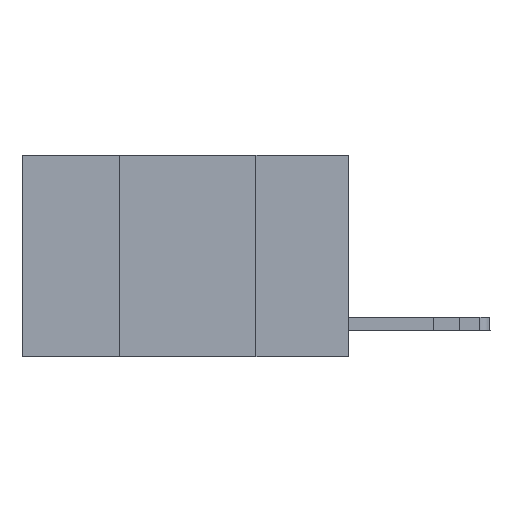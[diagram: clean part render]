
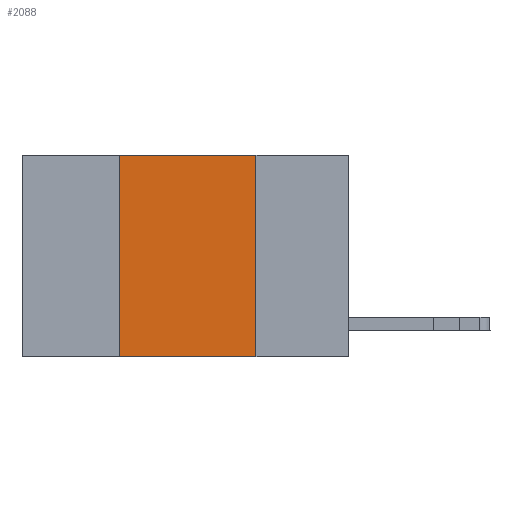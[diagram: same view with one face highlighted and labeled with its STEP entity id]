
A CAD part, left-side view. The second image highlights one B-rep face of the part: STEP entity #2088.
In plain terms, the highlighted planar face has unit normal (-1, 0, 0).
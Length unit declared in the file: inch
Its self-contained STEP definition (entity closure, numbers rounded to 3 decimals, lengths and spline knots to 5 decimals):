
#163 = DIRECTION ( 'NONE',  ( 0., 0., -1. ) ) ;
#490 = CARTESIAN_POINT ( 'NONE',  ( 0., 0.17, 0. ) ) ;
#843 = EDGE_CURVE ( 'NONE', #8674, #4050, #1412, .T. ) ;
#1412 = LINE ( 'NONE', #15500, #8013 ) ;
#1694 = CARTESIAN_POINT ( 'NONE',  ( 0., 0.42, -0.37 ) ) ;
#1748 = CARTESIAN_POINT ( 'NONE',  ( 0., 0.17, -0.37 ) ) ;
#2088 = ADVANCED_FACE ( 'NONE', ( #2604 ), #5808, .F. ) ;
#2604 = FACE_OUTER_BOUND ( 'NONE', #7482, .T. ) ;
#3079 = VECTOR ( 'NONE', #10672, 39.37008 ) ;
#3495 = EDGE_CURVE ( 'NONE', #8115, #10395, #9138, .T. ) ;
#4050 = VERTEX_POINT ( 'NONE', #14854 ) ;
#5767 = DIRECTION ( 'NONE',  ( 0., 0., -1. ) ) ;
#5770 = DIRECTION ( 'NONE',  ( 1., 0., 0. ) ) ;
#5808 = PLANE ( 'NONE',  #12335 ) ;
#5872 = CARTESIAN_POINT ( 'NONE',  ( 0., 0.6, 0. ) ) ;
#6030 = ORIENTED_EDGE ( 'NONE', *, *, #16099, .F. ) ;
#7482 = EDGE_LOOP ( 'NONE', ( #8717, #6030, #15037, #14268 ) ) ;
#7923 = LINE ( 'NONE', #14038, #13511 ) ;
#8013 = VECTOR ( 'NONE', #15484, 39.37008 ) ;
#8115 = VERTEX_POINT ( 'NONE', #12371 ) ;
#8674 = VERTEX_POINT ( 'NONE', #1694 ) ;
#8717 = ORIENTED_EDGE ( 'NONE', *, *, #3495, .F. ) ;
#9014 = DIRECTION ( 'NONE',  ( 0., -1., 0. ) ) ;
#9138 = LINE ( 'NONE', #490, #15433 ) ;
#10050 = LINE ( 'NONE', #11964, #3079 ) ;
#10395 = VERTEX_POINT ( 'NONE', #1748 ) ;
#10672 = DIRECTION ( 'NONE',  ( 0., -1., 0. ) ) ;
#11964 = CARTESIAN_POINT ( 'NONE',  ( 0., 0.6, -0.37 ) ) ;
#12335 = AXIS2_PLACEMENT_3D ( 'NONE', #5872, #5770, #5767 ) ;
#12371 = CARTESIAN_POINT ( 'NONE',  ( 0., 0.17, 0. ) ) ;
#13379 = EDGE_CURVE ( 'NONE', #8674, #10395, #10050, .T. ) ;
#13511 = VECTOR ( 'NONE', #9014, 39.37008 ) ;
#14038 = CARTESIAN_POINT ( 'NONE',  ( 0., 0.6, 0. ) ) ;
#14268 = ORIENTED_EDGE ( 'NONE', *, *, #13379, .T. ) ;
#14854 = CARTESIAN_POINT ( 'NONE',  ( 0., 0.42, 0. ) ) ;
#15037 = ORIENTED_EDGE ( 'NONE', *, *, #843, .F. ) ;
#15433 = VECTOR ( 'NONE', #163, 39.37008 ) ;
#15484 = DIRECTION ( 'NONE',  ( 0., 0., 1. ) ) ;
#15500 = CARTESIAN_POINT ( 'NONE',  ( 0., 0.42, 0. ) ) ;
#16099 = EDGE_CURVE ( 'NONE', #4050, #8115, #7923, .T. ) ;
